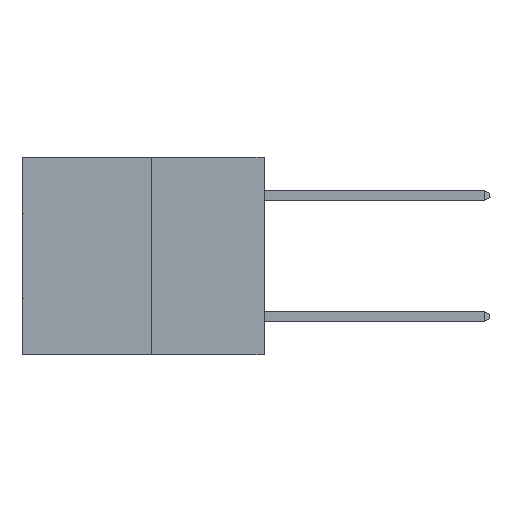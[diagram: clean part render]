
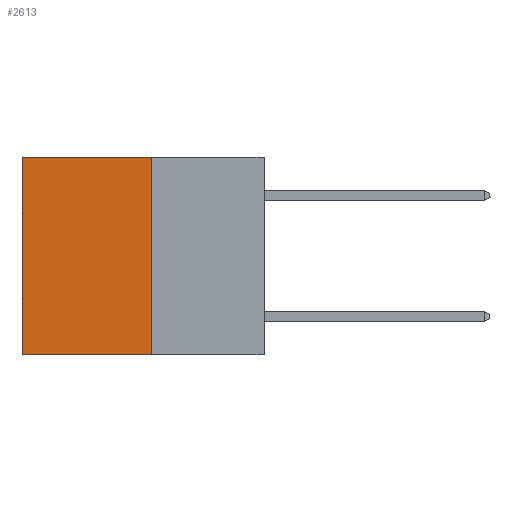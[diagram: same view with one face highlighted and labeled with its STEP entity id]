
A CAD part, left-side view. The second image highlights one B-rep face of the part: STEP entity #2613.
In plain terms, the highlighted planar face has unit normal (-1, 0, 0).
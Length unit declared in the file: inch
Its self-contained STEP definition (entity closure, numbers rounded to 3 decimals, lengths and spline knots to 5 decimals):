
#449 = VERTEX_POINT ( 'NONE', #11217 ) ;
#2381 = ORIENTED_EDGE ( 'NONE', *, *, #22850, .F. ) ;
#2613 = ADVANCED_FACE ( 'NONE', ( #30742 ), #18447, .F. ) ;
#2646 = AXIS2_PLACEMENT_3D ( 'NONE', #23142, #14090, #3861 ) ;
#2871 = VECTOR ( 'NONE', #18010, 39.37008 ) ;
#3263 = VECTOR ( 'NONE', #28976, 39.37008 ) ;
#3861 = DIRECTION ( 'NONE',  ( 0., 0., -1. ) ) ;
#5277 = DIRECTION ( 'NONE',  ( 0., 0., -1. ) ) ;
#7562 = CARTESIAN_POINT ( 'NONE',  ( 0.3165, 0.6, -0.49 ) ) ;
#8333 = CARTESIAN_POINT ( 'NONE',  ( 0.3165, 0.28, 0. ) ) ;
#9226 = VERTEX_POINT ( 'NONE', #18858 ) ;
#9466 = VECTOR ( 'NONE', #5277, 39.37008 ) ;
#10464 = CARTESIAN_POINT ( 'NONE',  ( 0.3165, 0.28, -0.49 ) ) ;
#11217 = CARTESIAN_POINT ( 'NONE',  ( 0.3165, 0.6, -0.49 ) ) ;
#11403 = EDGE_CURVE ( 'NONE', #23047, #449, #16559, .T. ) ;
#11429 = LINE ( 'NONE', #8333, #2871 ) ;
#14090 = DIRECTION ( 'NONE',  ( 1., 0., 0. ) ) ;
#15103 = VERTEX_POINT ( 'NONE', #29084 ) ;
#16559 = LINE ( 'NONE', #10464, #23202 ) ;
#18010 = DIRECTION ( 'NONE',  ( 0., 1., 0. ) ) ;
#18447 = PLANE ( 'NONE',  #2646 ) ;
#18858 = CARTESIAN_POINT ( 'NONE',  ( 0.3165, 0.28, 0. ) ) ;
#22850 = EDGE_CURVE ( 'NONE', #9226, #23047, #29810, .T. ) ;
#23047 = VERTEX_POINT ( 'NONE', #29979 ) ;
#23142 = CARTESIAN_POINT ( 'NONE',  ( 0.3165, 0.28, -0.49 ) ) ;
#23153 = ORIENTED_EDGE ( 'NONE', *, *, #31116, .T. ) ;
#23202 = VECTOR ( 'NONE', #30478, 39.37008 ) ;
#24252 = ORIENTED_EDGE ( 'NONE', *, *, #11403, .F. ) ;
#27167 = EDGE_LOOP ( 'NONE', ( #29411, #24252, #2381, #23153 ) ) ;
#28976 = DIRECTION ( 'NONE',  ( 0., 0., -1. ) ) ;
#29084 = CARTESIAN_POINT ( 'NONE',  ( 0.3165, 0.6, 0. ) ) ;
#29411 = ORIENTED_EDGE ( 'NONE', *, *, #31734, .T. ) ;
#29810 = LINE ( 'NONE', #31342, #3263 ) ;
#29979 = CARTESIAN_POINT ( 'NONE',  ( 0.3165, 0.28, -0.49 ) ) ;
#30478 = DIRECTION ( 'NONE',  ( 0., 1., 0. ) ) ;
#30742 = FACE_OUTER_BOUND ( 'NONE', #27167, .T. ) ;
#30866 = LINE ( 'NONE', #7562, #9466 ) ;
#31116 = EDGE_CURVE ( 'NONE', #9226, #15103, #11429, .T. ) ;
#31342 = CARTESIAN_POINT ( 'NONE',  ( 0.3165, 0.28, -0.49 ) ) ;
#31734 = EDGE_CURVE ( 'NONE', #15103, #449, #30866, .T. ) ;
